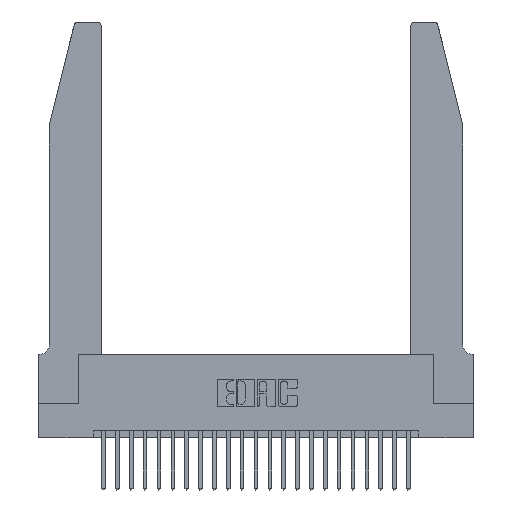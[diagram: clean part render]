
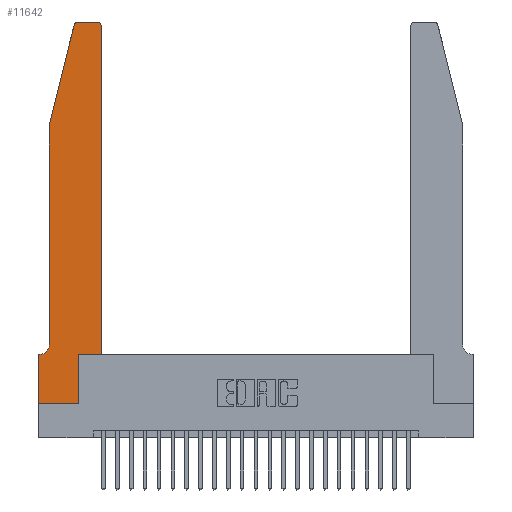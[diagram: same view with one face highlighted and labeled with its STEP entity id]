
A CAD part, top view. The second image highlights one B-rep face of the part: STEP entity #11642.
In plain terms, the highlighted planar face has unit normal (0, 0, 1).
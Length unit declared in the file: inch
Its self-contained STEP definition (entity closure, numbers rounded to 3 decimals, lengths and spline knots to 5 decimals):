
#706 = VERTEX_POINT ( 'NONE', #20041 ) ;
#1190 = VERTEX_POINT ( 'NONE', #18489 ) ;
#1303 = CARTESIAN_POINT ( 'NONE',  ( 0., 0., 0.37 ) ) ;
#1333 = CIRCLE ( 'NONE', #18472, 0.07 ) ;
#1449 = EDGE_CURVE ( 'NONE', #3256, #10817, #3499, .T. ) ;
#1577 = VECTOR ( 'NONE', #17726, 39.37008 ) ;
#1588 = EDGE_CURVE ( 'NONE', #10817, #706, #1333, .T. ) ;
#1713 = VECTOR ( 'NONE', #19574, 39.37008 ) ;
#1844 = EDGE_CURVE ( 'NONE', #6660, #1190, #4680, .T. ) ;
#1914 = ORIENTED_EDGE ( 'NONE', *, *, #20909, .T. ) ;
#1993 = AXIS2_PLACEMENT_3D ( 'NONE', #15204, #3152, #22806 ) ;
#2002 = LINE ( 'NONE', #13109, #1713 ) ;
#2844 = VECTOR ( 'NONE', #22465, 39.37008 ) ;
#3152 = DIRECTION ( 'NONE',  ( 0., 0., 1. ) ) ;
#3256 = VERTEX_POINT ( 'NONE', #22064 ) ;
#3499 = LINE ( 'NONE', #6854, #9297 ) ;
#3531 = DIRECTION ( 'NONE',  ( 0., -1., 0. ) ) ;
#4680 = LINE ( 'NONE', #18396, #2844 ) ;
#4842 = VECTOR ( 'NONE', #16674, 39.37008 ) ;
#5366 = VECTOR ( 'NONE', #18829, 39.37008 ) ;
#5671 = VERTEX_POINT ( 'NONE', #8847 ) ;
#5792 = EDGE_CURVE ( 'NONE', #6257, #20932, #19233, .T. ) ;
#6257 = VERTEX_POINT ( 'NONE', #7639 ) ;
#6311 = CARTESIAN_POINT ( 'NONE',  ( 0., 0.35, 0.37 ) ) ;
#6623 = DIRECTION ( 'NONE',  ( -0.239, -0.971, 0. ) ) ;
#6660 = VERTEX_POINT ( 'NONE', #7763 ) ;
#6705 = VERTEX_POINT ( 'NONE', #13318 ) ;
#6854 = CARTESIAN_POINT ( 'NONE',  ( 0.0755, 2., 0.37 ) ) ;
#7545 = EDGE_CURVE ( 'NONE', #706, #14573, #22091, .T. ) ;
#7639 = CARTESIAN_POINT ( 'NONE',  ( 0.4505, 2.72, 0.37 ) ) ;
#7763 = CARTESIAN_POINT ( 'NONE',  ( 0.2865, 0.35, 0.37 ) ) ;
#8138 = CIRCLE ( 'NONE', #12928, 0.03 ) ;
#8162 = ORIENTED_EDGE ( 'NONE', *, *, #1449, .T. ) ;
#8454 = LINE ( 'NONE', #8826, #19832 ) ;
#8826 = CARTESIAN_POINT ( 'NONE',  ( 0.4505, 0.35, 0.37 ) ) ;
#8847 = CARTESIAN_POINT ( 'NONE',  ( 0.284, 2.75, 0.37 ) ) ;
#9012 = ORIENTED_EDGE ( 'NONE', *, *, #1844, .T. ) ;
#9065 = EDGE_CURVE ( 'NONE', #16989, #6705, #21727, .T. ) ;
#9297 = VECTOR ( 'NONE', #3531, 39.37008 ) ;
#9868 = FACE_OUTER_BOUND ( 'NONE', #14742, .T. ) ;
#10817 = VERTEX_POINT ( 'NONE', #21939 ) ;
#10823 = CARTESIAN_POINT ( 'NONE',  ( 0., 0.35, 0.37 ) ) ;
#11642 = ADVANCED_FACE ( 'NONE', ( #9868 ), #12288, .T. ) ;
#11887 = ORIENTED_EDGE ( 'NONE', *, *, #22850, .T. ) ;
#11908 = DIRECTION ( 'NONE',  ( 1., 0., 0. ) ) ;
#11985 = VERTEX_POINT ( 'NONE', #22046 ) ;
#12288 = PLANE ( 'NONE',  #18820 ) ;
#12857 = CARTESIAN_POINT ( 'NONE',  ( 0.2605, 2.75, 0.37 ) ) ;
#12928 = AXIS2_PLACEMENT_3D ( 'NONE', #23692, #23058, #11908 ) ;
#13109 = CARTESIAN_POINT ( 'NONE',  ( 0.2865, 0.35, 0.37 ) ) ;
#13203 = ORIENTED_EDGE ( 'NONE', *, *, #14089, .T. ) ;
#13318 = CARTESIAN_POINT ( 'NONE',  ( 0.2865, 0., 0.37 ) ) ;
#13634 = ORIENTED_EDGE ( 'NONE', *, *, #22692, .T. ) ;
#13745 = DIRECTION ( 'NONE',  ( -1., 0., 0. ) ) ;
#14089 = EDGE_CURVE ( 'NONE', #11985, #3256, #21562, .T. ) ;
#14573 = VERTEX_POINT ( 'NONE', #10823 ) ;
#14585 = ORIENTED_EDGE ( 'NONE', *, *, #7545, .T. ) ;
#14625 = VECTOR ( 'NONE', #19890, 39.37008 ) ;
#14742 = EDGE_LOOP ( 'NONE', ( #13634, #19206, #13203, #8162, #17562, #14585, #17870, #19721, #11887, #9012, #1914, #22808 ) ) ;
#14771 = DIRECTION ( 'NONE',  ( 0., 1., 0. ) ) ;
#15204 = CARTESIAN_POINT ( 'NONE',  ( 0.4205, 2.72, 0.37 ) ) ;
#16266 = CARTESIAN_POINT ( 'NONE',  ( 0., 0., 0.37 ) ) ;
#16674 = DIRECTION ( 'NONE',  ( 1., 0., 0. ) ) ;
#16989 = VERTEX_POINT ( 'NONE', #1303 ) ;
#17562 = ORIENTED_EDGE ( 'NONE', *, *, #1588, .T. ) ;
#17720 = DIRECTION ( 'NONE',  ( 0., 0., -1. ) ) ;
#17726 = DIRECTION ( 'NONE',  ( -1., 0., 0. ) ) ;
#17870 = ORIENTED_EDGE ( 'NONE', *, *, #21217, .T. ) ;
#18396 = CARTESIAN_POINT ( 'NONE',  ( 0.4505, 0.35, 0.37 ) ) ;
#18461 = VECTOR ( 'NONE', #6623, 39.37008 ) ;
#18472 = AXIS2_PLACEMENT_3D ( 'NONE', #23428, #17720, #13745 ) ;
#18489 = CARTESIAN_POINT ( 'NONE',  ( 0.4505, 0.35, 0.37 ) ) ;
#18574 = CARTESIAN_POINT ( 'NONE',  ( 0., 0., 0.37 ) ) ;
#18631 = CARTESIAN_POINT ( 'NONE',  ( 0.4205, 2.75, 0.37 ) ) ;
#18820 = AXIS2_PLACEMENT_3D ( 'NONE', #6311, #21783, #21931 ) ;
#18829 = DIRECTION ( 'NONE',  ( -1., 0., 0. ) ) ;
#19206 = ORIENTED_EDGE ( 'NONE', *, *, #21058, .T. ) ;
#19233 = CIRCLE ( 'NONE', #1993, 0.03 ) ;
#19574 = DIRECTION ( 'NONE',  ( 0., 1., 0. ) ) ;
#19721 = ORIENTED_EDGE ( 'NONE', *, *, #9065, .T. ) ;
#19832 = VECTOR ( 'NONE', #14771, 39.37008 ) ;
#19857 = LINE ( 'NONE', #16266, #14625 ) ;
#19890 = DIRECTION ( 'NONE',  ( 0., -1., 0. ) ) ;
#20041 = CARTESIAN_POINT ( 'NONE',  ( 0.0055, 0.35, 0.37 ) ) ;
#20909 = EDGE_CURVE ( 'NONE', #1190, #6257, #8454, .T. ) ;
#20932 = VERTEX_POINT ( 'NONE', #18631 ) ;
#21021 = LINE ( 'NONE', #12857, #5366 ) ;
#21058 = EDGE_CURVE ( 'NONE', #5671, #11985, #8138, .T. ) ;
#21217 = EDGE_CURVE ( 'NONE', #14573, #16989, #19857, .T. ) ;
#21286 = CARTESIAN_POINT ( 'NONE',  ( 0.0755, 0.35, 0.37 ) ) ;
#21562 = LINE ( 'NONE', #24122, #18461 ) ;
#21727 = LINE ( 'NONE', #18574, #4842 ) ;
#21783 = DIRECTION ( 'NONE',  ( 0., 0., 1. ) ) ;
#21931 = DIRECTION ( 'NONE',  ( 1., 0., 0. ) ) ;
#21939 = CARTESIAN_POINT ( 'NONE',  ( 0.0755, 0.42, 0.37 ) ) ;
#22046 = CARTESIAN_POINT ( 'NONE',  ( 0.25487, 2.72718, 0.37 ) ) ;
#22064 = CARTESIAN_POINT ( 'NONE',  ( 0.0755, 2., 0.37 ) ) ;
#22091 = LINE ( 'NONE', #21286, #1577 ) ;
#22465 = DIRECTION ( 'NONE',  ( 1., 0., 0. ) ) ;
#22692 = EDGE_CURVE ( 'NONE', #20932, #5671, #21021, .T. ) ;
#22806 = DIRECTION ( 'NONE',  ( 1., 0., 0. ) ) ;
#22808 = ORIENTED_EDGE ( 'NONE', *, *, #5792, .T. ) ;
#22850 = EDGE_CURVE ( 'NONE', #6705, #6660, #2002, .T. ) ;
#23058 = DIRECTION ( 'NONE',  ( 0., 0., 1. ) ) ;
#23428 = CARTESIAN_POINT ( 'NONE',  ( 0.0055, 0.42, 0.37 ) ) ;
#23692 = CARTESIAN_POINT ( 'NONE',  ( 0.284, 2.72, 0.37 ) ) ;
#24122 = CARTESIAN_POINT ( 'NONE',  ( 0.0755, 2., 0.37 ) ) ;
